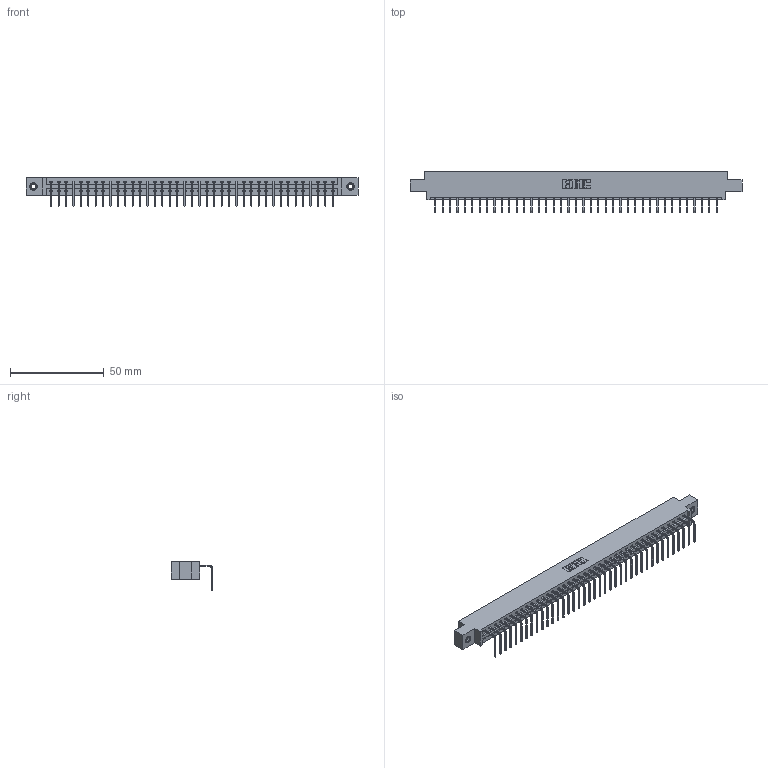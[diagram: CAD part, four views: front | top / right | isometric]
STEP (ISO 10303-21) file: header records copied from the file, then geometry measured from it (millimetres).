
FILE_DESCRIPTION (( 'STEP AP203' ), '1' );
FILE_NAME ('337-039-558-607.STEP', '2018-08-08T08:14:43', ( '' ), ( '' ), 'SwSTEP 2.0', 'SolidWorks 2016', '' );
FILE_SCHEMA (( 'CONFIG_CONTROL_DESIGN' ));
Length unit declared in the file: inch
Products named in the file (4): 337 Part_0.170 Offset - 0.156 Dia-TI; 345-292-001_558 Tail - 2; 345-250-001_345-250-005-103; 337-039-558-607
Assembly tree (42 placements, depth 2):
  337-039-558-607
    337 Part_0.170 Offset - 0.156 Dia-TI
    345-292-001_558 Tail - 2  x39
    345-250-001_345-250-005-103  x2
Bounding box: 177.55 x 22.17 x 15.37 mm (x, y, z)
Volume: 18414.3 mm3; surface area: 19947.6 mm2
Topology: 42 solids, 42 shells, 2674 faces, 8025 edges, 5290 vertices
Faces by surface type: plane 1978, cylinder 680, cone 12, torus 4
Entity records: 30780 total; most frequent: CARTESIAN_POINT 5342, ORIENTED_EDGE 5310, DIRECTION 4535, EDGE_CURVE 2655, VECTOR 2507, LINE 2507, VERTEX_POINT 1764, AXIS2_PLACEMENT_3D 1014
